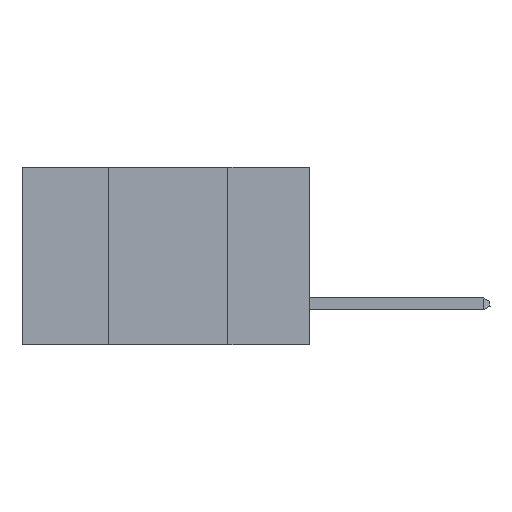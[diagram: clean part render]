
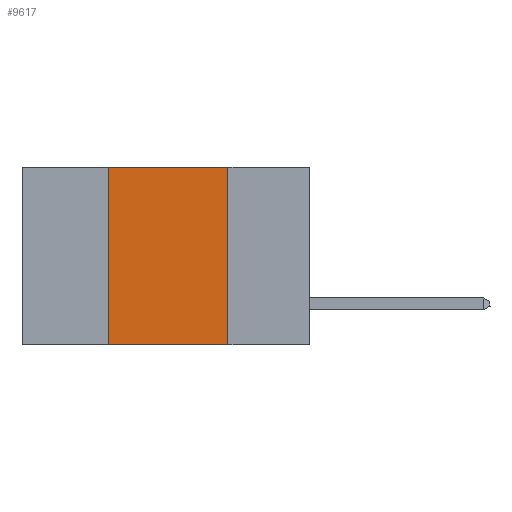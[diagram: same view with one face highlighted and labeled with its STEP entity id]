
A CAD part, left-side view. The second image highlights one B-rep face of the part: STEP entity #9617.
In plain terms, the highlighted planar face has unit normal (-1, 0, 0).
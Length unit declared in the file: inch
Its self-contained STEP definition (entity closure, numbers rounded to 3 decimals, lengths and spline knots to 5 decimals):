
#98 = CARTESIAN_POINT ( 'NONE',  ( 0., 0.6, -0.37 ) ) ;
#796 = VECTOR ( 'NONE', #7978, 39.37008 ) ;
#1133 = LINE ( 'NONE', #7746, #2522 ) ;
#1310 = LINE ( 'NONE', #98, #12615 ) ;
#2522 = VECTOR ( 'NONE', #4402, 39.37008 ) ;
#2988 = DIRECTION ( 'NONE',  ( 0., 0., -1. ) ) ;
#3118 = ORIENTED_EDGE ( 'NONE', *, *, #3864, .T. ) ;
#3864 = EDGE_CURVE ( 'NONE', #13772, #12901, #1310, .T. ) ;
#4398 = VECTOR ( 'NONE', #11089, 39.37008 ) ;
#4402 = DIRECTION ( 'NONE',  ( 0., 0., 1. ) ) ;
#4541 = CARTESIAN_POINT ( 'NONE',  ( 0., 0.17, 0. ) ) ;
#4847 = VERTEX_POINT ( 'NONE', #9499 ) ;
#5015 = EDGE_CURVE ( 'NONE', #4847, #12901, #12772, .T. ) ;
#5606 = DIRECTION ( 'NONE',  ( 0., -1., 0. ) ) ;
#6073 = CARTESIAN_POINT ( 'NONE',  ( 0., 0.42, -0.37 ) ) ;
#6202 = PLANE ( 'NONE',  #12900 ) ;
#7746 = CARTESIAN_POINT ( 'NONE',  ( 0., 0.42, 0. ) ) ;
#7789 = FACE_OUTER_BOUND ( 'NONE', #11181, .T. ) ;
#7978 = DIRECTION ( 'NONE',  ( 0., 0., -1. ) ) ;
#8138 = VERTEX_POINT ( 'NONE', #12426 ) ;
#9499 = CARTESIAN_POINT ( 'NONE',  ( 0., 0.17, 0. ) ) ;
#9617 = ADVANCED_FACE ( 'NONE', ( #7789 ), #6202, .F. ) ;
#9691 = DIRECTION ( 'NONE',  ( 1., 0., 0. ) ) ;
#9796 = ORIENTED_EDGE ( 'NONE', *, *, #11016, .F. ) ;
#10184 = LINE ( 'NONE', #12251, #4398 ) ;
#10495 = ORIENTED_EDGE ( 'NONE', *, *, #11690, .F. ) ;
#11016 = EDGE_CURVE ( 'NONE', #13772, #8138, #1133, .T. ) ;
#11089 = DIRECTION ( 'NONE',  ( 0., -1., 0. ) ) ;
#11181 = EDGE_LOOP ( 'NONE', ( #14141, #10495, #9796, #3118 ) ) ;
#11690 = EDGE_CURVE ( 'NONE', #8138, #4847, #10184, .T. ) ;
#12251 = CARTESIAN_POINT ( 'NONE',  ( 0., 0.6, 0. ) ) ;
#12426 = CARTESIAN_POINT ( 'NONE',  ( 0., 0.42, 0. ) ) ;
#12615 = VECTOR ( 'NONE', #5606, 39.37008 ) ;
#12772 = LINE ( 'NONE', #4541, #796 ) ;
#12900 = AXIS2_PLACEMENT_3D ( 'NONE', #12914, #9691, #2988 ) ;
#12901 = VERTEX_POINT ( 'NONE', #13302 ) ;
#12914 = CARTESIAN_POINT ( 'NONE',  ( 0., 0.6, 0. ) ) ;
#13302 = CARTESIAN_POINT ( 'NONE',  ( 0., 0.17, -0.37 ) ) ;
#13772 = VERTEX_POINT ( 'NONE', #6073 ) ;
#14141 = ORIENTED_EDGE ( 'NONE', *, *, #5015, .F. ) ;
